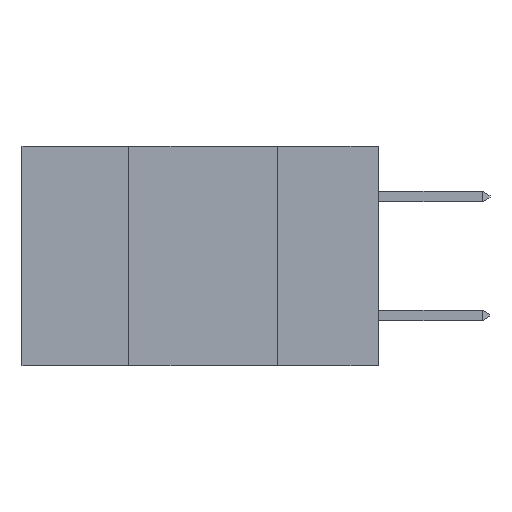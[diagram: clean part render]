
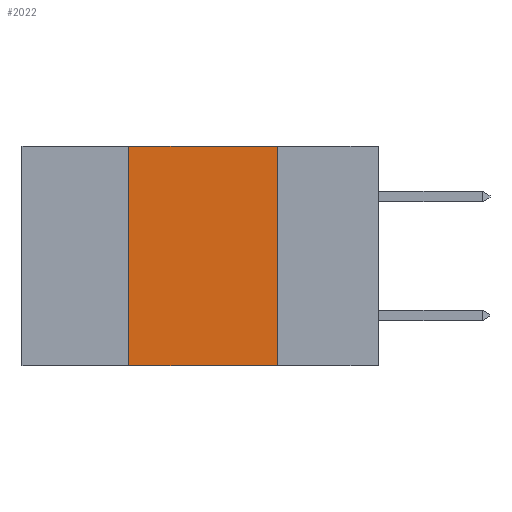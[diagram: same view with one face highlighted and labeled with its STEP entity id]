
A CAD part, left-side view. The second image highlights one B-rep face of the part: STEP entity #2022.
In plain terms, the highlighted planar face has unit normal (-1, 0, 0).
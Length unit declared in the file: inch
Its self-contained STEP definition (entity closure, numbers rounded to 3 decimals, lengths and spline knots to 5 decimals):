
#8 = LINE ( 'NONE', #10812, #11319 ) ;
#740 = VECTOR ( 'NONE', #4913, 39.37008 ) ;
#2009 = DIRECTION ( 'NONE',  ( 1., 0., 0. ) ) ;
#2022 = ADVANCED_FACE ( 'NONE', ( #11321 ), #11747, .F. ) ;
#2502 = DIRECTION ( 'NONE',  ( 0., 0., 1. ) ) ;
#2539 = CARTESIAN_POINT ( 'NONE',  ( 0., 0.42, 0. ) ) ;
#3261 = CARTESIAN_POINT ( 'NONE',  ( 0., 0.6, 0. ) ) ;
#3873 = ORIENTED_EDGE ( 'NONE', *, *, #11614, .T. ) ;
#4600 = EDGE_CURVE ( 'NONE', #11087, #5786, #9285, .T. ) ;
#4913 = DIRECTION ( 'NONE',  ( 0., -1., 0. ) ) ;
#5568 = CARTESIAN_POINT ( 'NONE',  ( 0., 0.17, -0.37 ) ) ;
#5757 = DIRECTION ( 'NONE',  ( 0., 0., -1. ) ) ;
#5786 = VERTEX_POINT ( 'NONE', #10095 ) ;
#6472 = VECTOR ( 'NONE', #2502, 39.37008 ) ;
#7158 = CARTESIAN_POINT ( 'NONE',  ( 0., 0.17, 0. ) ) ;
#7301 = EDGE_CURVE ( 'NONE', #11928, #11351, #10461, .T. ) ;
#9285 = LINE ( 'NONE', #2539, #6472 ) ;
#9367 = ORIENTED_EDGE ( 'NONE', *, *, #4600, .F. ) ;
#9727 = EDGE_LOOP ( 'NONE', ( #10456, #10768, #9367, #3873 ) ) ;
#10095 = CARTESIAN_POINT ( 'NONE',  ( 0., 0.42, 0. ) ) ;
#10456 = ORIENTED_EDGE ( 'NONE', *, *, #7301, .F. ) ;
#10461 = LINE ( 'NONE', #13004, #12847 ) ;
#10768 = ORIENTED_EDGE ( 'NONE', *, *, #12270, .F. ) ;
#10812 = CARTESIAN_POINT ( 'NONE',  ( 0., 0.6, 0. ) ) ;
#11087 = VERTEX_POINT ( 'NONE', #11275 ) ;
#11275 = CARTESIAN_POINT ( 'NONE',  ( 0., 0.42, -0.37 ) ) ;
#11319 = VECTOR ( 'NONE', #11825, 39.37008 ) ;
#11321 = FACE_OUTER_BOUND ( 'NONE', #9727, .T. ) ;
#11351 = VERTEX_POINT ( 'NONE', #5568 ) ;
#11614 = EDGE_CURVE ( 'NONE', #11087, #11351, #12265, .T. ) ;
#11619 = AXIS2_PLACEMENT_3D ( 'NONE', #3261, #2009, #5757 ) ;
#11747 = PLANE ( 'NONE',  #11619 ) ;
#11825 = DIRECTION ( 'NONE',  ( 0., -1., 0. ) ) ;
#11928 = VERTEX_POINT ( 'NONE', #7158 ) ;
#12265 = LINE ( 'NONE', #13328, #740 ) ;
#12270 = EDGE_CURVE ( 'NONE', #5786, #11928, #8, .T. ) ;
#12847 = VECTOR ( 'NONE', #12989, 39.37008 ) ;
#12989 = DIRECTION ( 'NONE',  ( 0., 0., -1. ) ) ;
#13004 = CARTESIAN_POINT ( 'NONE',  ( 0., 0.17, 0. ) ) ;
#13328 = CARTESIAN_POINT ( 'NONE',  ( 0., 0.6, -0.37 ) ) ;
